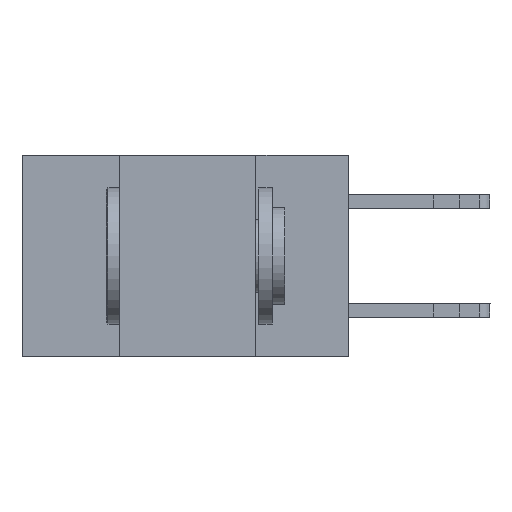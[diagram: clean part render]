
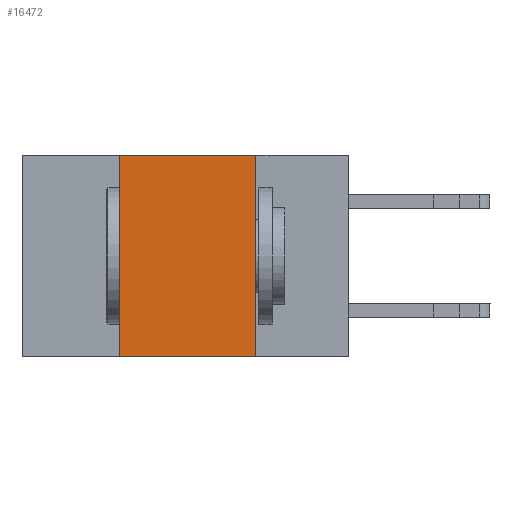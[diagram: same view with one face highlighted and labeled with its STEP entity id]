
A CAD part, left-side view. The second image highlights one B-rep face of the part: STEP entity #16472.
In plain terms, the highlighted planar face has unit normal (-1, 0, 0).
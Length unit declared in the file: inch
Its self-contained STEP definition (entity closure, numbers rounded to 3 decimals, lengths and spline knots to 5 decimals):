
#35 = FACE_OUTER_BOUND ( 'NONE', #24890, .T. ) ;
#769 = EDGE_CURVE ( 'NONE', #7338, #11596, #2082, .T. ) ;
#1372 = CARTESIAN_POINT ( 'NONE',  ( 0., 0.17, 0. ) ) ;
#2061 = CARTESIAN_POINT ( 'NONE',  ( 0., 0.6, 0. ) ) ;
#2082 = LINE ( 'NONE', #11527, #10266 ) ;
#2152 = PLANE ( 'NONE',  #15901 ) ;
#6365 = DIRECTION ( 'NONE',  ( 1., 0., 0. ) ) ;
#7104 = LINE ( 'NONE', #11224, #8118 ) ;
#7338 = VERTEX_POINT ( 'NONE', #11622 ) ;
#8118 = VECTOR ( 'NONE', #11516, 39.37008 ) ;
#9518 = ORIENTED_EDGE ( 'NONE', *, *, #25034, .F. ) ;
#9711 = VERTEX_POINT ( 'NONE', #25022 ) ;
#10266 = VECTOR ( 'NONE', #15698, 39.37008 ) ;
#10733 = DIRECTION ( 'NONE',  ( 0., 0., -1. ) ) ;
#10735 = CARTESIAN_POINT ( 'NONE',  ( 0., 0.17, 0. ) ) ;
#10759 = VECTOR ( 'NONE', #27494, 39.37008 ) ;
#11224 = CARTESIAN_POINT ( 'NONE',  ( 0., 0.6, 0. ) ) ;
#11516 = DIRECTION ( 'NONE',  ( 0., -1., 0. ) ) ;
#11527 = CARTESIAN_POINT ( 'NONE',  ( 0., 0.42, 0. ) ) ;
#11596 = VERTEX_POINT ( 'NONE', #15419 ) ;
#11622 = CARTESIAN_POINT ( 'NONE',  ( 0., 0.42, -0.37 ) ) ;
#12173 = VECTOR ( 'NONE', #25754, 39.37008 ) ;
#12928 = EDGE_CURVE ( 'NONE', #11596, #26632, #7104, .T. ) ;
#15419 = CARTESIAN_POINT ( 'NONE',  ( 0., 0.42, 0. ) ) ;
#15698 = DIRECTION ( 'NONE',  ( 0., 0., 1. ) ) ;
#15783 = ORIENTED_EDGE ( 'NONE', *, *, #12928, .F. ) ;
#15901 = AXIS2_PLACEMENT_3D ( 'NONE', #2061, #6365, #10733 ) ;
#16472 = ADVANCED_FACE ( 'NONE', ( #35 ), #2152, .F. ) ;
#16507 = LINE ( 'NONE', #1372, #10759 ) ;
#17032 = CARTESIAN_POINT ( 'NONE',  ( 0., 0.6, -0.37 ) ) ;
#17890 = LINE ( 'NONE', #17032, #12173 ) ;
#21159 = ORIENTED_EDGE ( 'NONE', *, *, #21945, .T. ) ;
#21945 = EDGE_CURVE ( 'NONE', #7338, #9711, #17890, .T. ) ;
#24890 = EDGE_LOOP ( 'NONE', ( #9518, #15783, #25512, #21159 ) ) ;
#25022 = CARTESIAN_POINT ( 'NONE',  ( 0., 0.17, -0.37 ) ) ;
#25034 = EDGE_CURVE ( 'NONE', #26632, #9711, #16507, .T. ) ;
#25512 = ORIENTED_EDGE ( 'NONE', *, *, #769, .F. ) ;
#25754 = DIRECTION ( 'NONE',  ( 0., -1., 0. ) ) ;
#26632 = VERTEX_POINT ( 'NONE', #10735 ) ;
#27494 = DIRECTION ( 'NONE',  ( 0., 0., -1. ) ) ;
